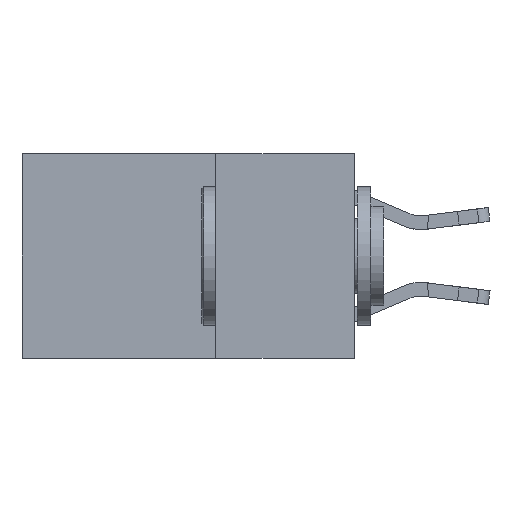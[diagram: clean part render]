
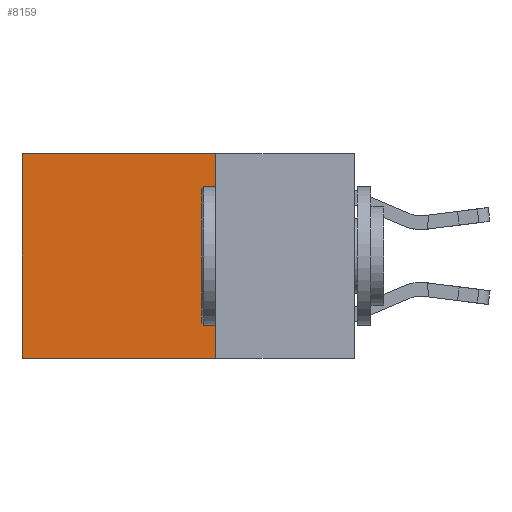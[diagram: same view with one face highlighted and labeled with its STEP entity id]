
A CAD part, left-side view. The second image highlights one B-rep face of the part: STEP entity #8159.
In plain terms, the highlighted planar face has unit normal (-1, 0, 0).
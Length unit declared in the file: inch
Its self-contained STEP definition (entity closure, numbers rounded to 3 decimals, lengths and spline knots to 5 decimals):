
#68 = VECTOR ( 'NONE', #5469, 39.37008 ) ;
#201 = FACE_OUTER_BOUND ( 'NONE', #2987, .T. ) ;
#444 = DIRECTION ( 'NONE',  ( 1., 0., 0. ) ) ;
#1342 = VECTOR ( 'NONE', #15420, 39.37008 ) ;
#1377 = EDGE_CURVE ( 'NONE', #14300, #3882, #8942, .T. ) ;
#2987 = EDGE_LOOP ( 'NONE', ( #10152, #14915, #7226, #10864 ) ) ;
#3870 = CARTESIAN_POINT ( 'NONE',  ( 0.2625, 0.25, 0. ) ) ;
#3882 = VERTEX_POINT ( 'NONE', #5405 ) ;
#5140 = LINE ( 'NONE', #11231, #1342 ) ;
#5405 = CARTESIAN_POINT ( 'NONE',  ( 0.2625, 0.6, -0.37 ) ) ;
#5469 = DIRECTION ( 'NONE',  ( 0., 1., 0. ) ) ;
#5623 = VERTEX_POINT ( 'NONE', #7652 ) ;
#7226 = ORIENTED_EDGE ( 'NONE', *, *, #15333, .F. ) ;
#7516 = PLANE ( 'NONE',  #12279 ) ;
#7652 = CARTESIAN_POINT ( 'NONE',  ( 0.2625, 0.25, 0. ) ) ;
#7860 = DIRECTION ( 'NONE',  ( 0., 0., -1. ) ) ;
#7944 = CARTESIAN_POINT ( 'NONE',  ( 0.2625, 0.6, 0. ) ) ;
#8159 = ADVANCED_FACE ( 'NONE', ( #201 ), #7516, .F. ) ;
#8500 = VECTOR ( 'NONE', #12148, 39.37008 ) ;
#8523 = VECTOR ( 'NONE', #7860, 39.37008 ) ;
#8942 = LINE ( 'NONE', #7944, #8523 ) ;
#10152 = ORIENTED_EDGE ( 'NONE', *, *, #1377, .T. ) ;
#10263 = DIRECTION ( 'NONE',  ( 0., 0., -1. ) ) ;
#10864 = ORIENTED_EDGE ( 'NONE', *, *, #12350, .T. ) ;
#11003 = CARTESIAN_POINT ( 'NONE',  ( 0.2625, 0.6, 0. ) ) ;
#11231 = CARTESIAN_POINT ( 'NONE',  ( 0.2625, 0.25, 0. ) ) ;
#11260 = LINE ( 'NONE', #15124, #68 ) ;
#12148 = DIRECTION ( 'NONE',  ( 0., 1., 0. ) ) ;
#12279 = AXIS2_PLACEMENT_3D ( 'NONE', #17147, #444, #10263 ) ;
#12350 = EDGE_CURVE ( 'NONE', #5623, #14300, #15829, .T. ) ;
#12428 = EDGE_CURVE ( 'NONE', #15937, #3882, #11260, .T. ) ;
#13946 = CARTESIAN_POINT ( 'NONE',  ( 0.2625, 0.25, -0.37 ) ) ;
#14300 = VERTEX_POINT ( 'NONE', #11003 ) ;
#14915 = ORIENTED_EDGE ( 'NONE', *, *, #12428, .F. ) ;
#15124 = CARTESIAN_POINT ( 'NONE',  ( 0.2625, 0.25, -0.37 ) ) ;
#15333 = EDGE_CURVE ( 'NONE', #5623, #15937, #5140, .T. ) ;
#15420 = DIRECTION ( 'NONE',  ( 0., 0., -1. ) ) ;
#15829 = LINE ( 'NONE', #3870, #8500 ) ;
#15937 = VERTEX_POINT ( 'NONE', #13946 ) ;
#17147 = CARTESIAN_POINT ( 'NONE',  ( 0.2625, 0.25, 0. ) ) ;
